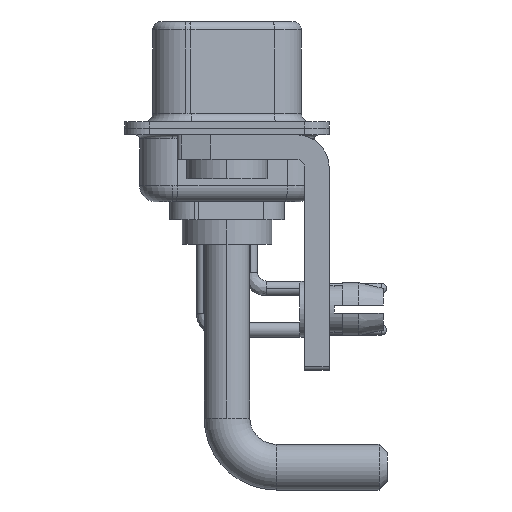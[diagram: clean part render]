
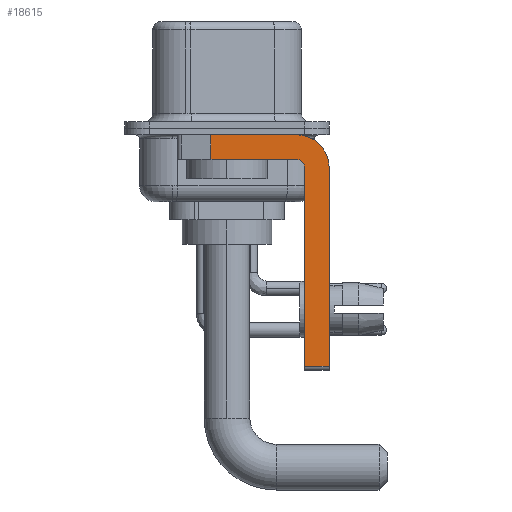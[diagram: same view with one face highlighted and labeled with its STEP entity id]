
A CAD part, left-side view. The second image highlights one B-rep face of the part: STEP entity #18615.
In plain terms, the highlighted planar face has unit normal (-1, 0, 0).
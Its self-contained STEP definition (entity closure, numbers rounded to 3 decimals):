
#31 = CIRCLE ( 'NONE', #7088, 2. ) ;
#266 = LINE ( 'NONE', #15068, #31028 ) ;
#1104 = LINE ( 'NONE', #5683, #25639 ) ;
#1547 = CARTESIAN_POINT ( 'NONE',  ( -2.9, -6.25, -2.4 ) ) ;
#2084 = ORIENTED_EDGE ( 'NONE', *, *, #31019, .T. ) ;
#2318 = DIRECTION ( 'NONE',  ( 0., 0., -1. ) ) ;
#3242 = DIRECTION ( 'NONE',  ( 0., 0., 1. ) ) ;
#3774 = VECTOR ( 'NONE', #17160, 1000. ) ;
#3948 = CARTESIAN_POINT ( 'NONE',  ( -2.9, -4.25, -2.4 ) ) ;
#4085 = ORIENTED_EDGE ( 'NONE', *, *, #9180, .F. ) ;
#5086 = LINE ( 'NONE', #9816, #18536 ) ;
#5683 = CARTESIAN_POINT ( 'NONE',  ( -2.9, -4.75, -14.8 ) ) ;
#6186 = EDGE_CURVE ( 'NONE', #23608, #22047, #266, .T. ) ;
#6441 = PLANE ( 'NONE',  #25443 ) ;
#6737 = VERTEX_POINT ( 'NONE', #29337 ) ;
#6742 = FACE_OUTER_BOUND ( 'NONE', #27455, .T. ) ;
#7088 = AXIS2_PLACEMENT_3D ( 'NONE', #3948, #15284, #20465 ) ;
#7280 = EDGE_CURVE ( 'NONE', #26737, #8446, #5086, .T. ) ;
#8320 = CARTESIAN_POINT ( 'NONE',  ( -2.9, 0.978, -1.9 ) ) ;
#8354 = CARTESIAN_POINT ( 'NONE',  ( -2.9, -4.75, -14.55 ) ) ;
#8446 = VERTEX_POINT ( 'NONE', #28208 ) ;
#9180 = EDGE_CURVE ( 'NONE', #26737, #20554, #1104, .T. ) ;
#9816 = CARTESIAN_POINT ( 'NONE',  ( -2.9, -4.25, -14.55 ) ) ;
#10324 = CARTESIAN_POINT ( 'NONE',  ( -2.9, -4.25, -0.4 ) ) ;
#12038 = LINE ( 'NONE', #26469, #24812 ) ;
#12254 = DIRECTION ( 'NONE',  ( 0., -1., 0. ) ) ;
#12763 = DIRECTION ( 'NONE',  ( 0., 0., 1. ) ) ;
#14424 = CARTESIAN_POINT ( 'NONE',  ( -2.9, -4.75, -2.4 ) ) ;
#14529 = ORIENTED_EDGE ( 'NONE', *, *, #7280, .T. ) ;
#14686 = DIRECTION ( 'NONE',  ( 0., -1., 0. ) ) ;
#14778 = EDGE_CURVE ( 'NONE', #6737, #28372, #25000, .T. ) ;
#15068 = CARTESIAN_POINT ( 'NONE',  ( -2.9, 3., -0.4 ) ) ;
#15205 = CARTESIAN_POINT ( 'NONE',  ( -2.9, -4.25, -2.4 ) ) ;
#15284 = DIRECTION ( 'NONE',  ( 1., 0., 0. ) ) ;
#17160 = DIRECTION ( 'NONE',  ( 0., 1., 0. ) ) ;
#18070 = AXIS2_PLACEMENT_3D ( 'NONE', #15205, #24782, #3242 ) ;
#18448 = VERTEX_POINT ( 'NONE', #1547 ) ;
#18536 = VECTOR ( 'NONE', #14686, 1000. ) ;
#18615 = ADVANCED_FACE ( 'NONE', ( #6742 ), #6441, .F. ) ;
#18801 = CARTESIAN_POINT ( 'NONE',  ( -2.9, 0.978, -0.4 ) ) ;
#19205 = ORIENTED_EDGE ( 'NONE', *, *, #14778, .F. ) ;
#19277 = VECTOR ( 'NONE', #24615, 1000. ) ;
#20465 = DIRECTION ( 'NONE',  ( 0., 0., -1. ) ) ;
#20554 = VERTEX_POINT ( 'NONE', #14424 ) ;
#20606 = ORIENTED_EDGE ( 'NONE', *, *, #30707, .F. ) ;
#21361 = DIRECTION ( 'NONE',  ( 1., 0., 0. ) ) ;
#22047 = VERTEX_POINT ( 'NONE', #10324 ) ;
#22414 = LINE ( 'NONE', #22571, #19277 ) ;
#22571 = CARTESIAN_POINT ( 'NONE',  ( -2.9, -6.25, -2.4 ) ) ;
#23355 = EDGE_CURVE ( 'NONE', #20554, #6737, #30118, .T. ) ;
#23542 = ORIENTED_EDGE ( 'NONE', *, *, #26667, .F. ) ;
#23608 = VERTEX_POINT ( 'NONE', #18801 ) ;
#23875 = CARTESIAN_POINT ( 'NONE',  ( -2.9, -4.25, -2.4 ) ) ;
#24615 = DIRECTION ( 'NONE',  ( 0., 0., -1. ) ) ;
#24782 = DIRECTION ( 'NONE',  ( -1., 0., 0. ) ) ;
#24812 = VECTOR ( 'NONE', #31050, 1000. ) ;
#25000 = LINE ( 'NONE', #29415, #3774 ) ;
#25443 = AXIS2_PLACEMENT_3D ( 'NONE', #23875, #21361, #2318 ) ;
#25639 = VECTOR ( 'NONE', #12763, 1000. ) ;
#26469 = CARTESIAN_POINT ( 'NONE',  ( -2.9, 0.978, -1.9 ) ) ;
#26667 = EDGE_CURVE ( 'NONE', #22047, #18448, #31, .T. ) ;
#26737 = VERTEX_POINT ( 'NONE', #8354 ) ;
#27455 = EDGE_LOOP ( 'NONE', ( #30968, #2084, #19205, #29916, #4085, #14529, #20606, #23542 ) ) ;
#28208 = CARTESIAN_POINT ( 'NONE',  ( -2.9, -6.25, -14.55 ) ) ;
#28372 = VERTEX_POINT ( 'NONE', #8320 ) ;
#29337 = CARTESIAN_POINT ( 'NONE',  ( -2.9, -4.25, -1.9 ) ) ;
#29415 = CARTESIAN_POINT ( 'NONE',  ( -2.9, -4.25, -1.9 ) ) ;
#29916 = ORIENTED_EDGE ( 'NONE', *, *, #23355, .F. ) ;
#30118 = CIRCLE ( 'NONE', #18070, 0.5 ) ;
#30707 = EDGE_CURVE ( 'NONE', #18448, #8446, #22414, .T. ) ;
#30968 = ORIENTED_EDGE ( 'NONE', *, *, #6186, .F. ) ;
#31019 = EDGE_CURVE ( 'NONE', #23608, #28372, #12038, .T. ) ;
#31028 = VECTOR ( 'NONE', #12254, 1000. ) ;
#31050 = DIRECTION ( 'NONE',  ( 0., 0., -1. ) ) ;
